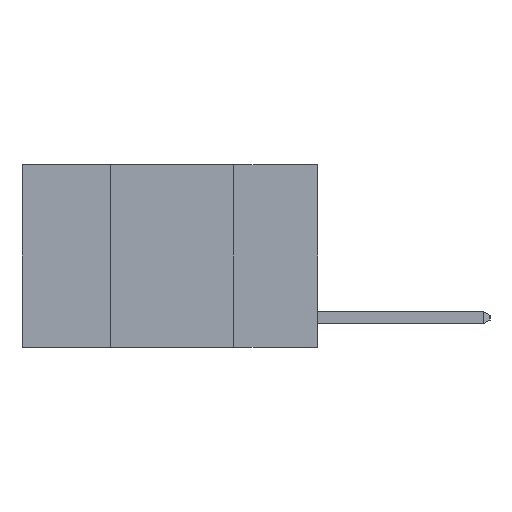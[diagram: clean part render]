
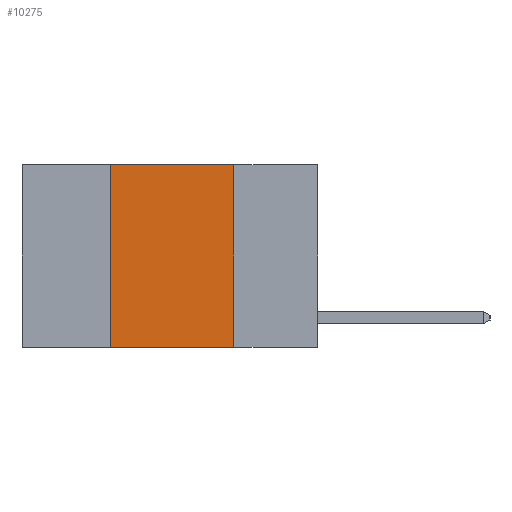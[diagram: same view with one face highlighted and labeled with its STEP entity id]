
A CAD part, left-side view. The second image highlights one B-rep face of the part: STEP entity #10275.
In plain terms, the highlighted planar face has unit normal (-1, 0, 0).
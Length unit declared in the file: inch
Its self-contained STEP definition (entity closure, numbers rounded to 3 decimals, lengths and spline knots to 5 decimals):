
#359 = DIRECTION ( 'NONE',  ( 0., 0., -1. ) ) ;
#1128 = DIRECTION ( 'NONE',  ( 0., -1., 0. ) ) ;
#1276 = LINE ( 'NONE', #9373, #3258 ) ;
#1300 = LINE ( 'NONE', #7426, #7578 ) ;
#1443 = ORIENTED_EDGE ( 'NONE', *, *, #9543, .F. ) ;
#1784 = LINE ( 'NONE', #6048, #2316 ) ;
#2316 = VECTOR ( 'NONE', #1128, 39.37008 ) ;
#2879 = CARTESIAN_POINT ( 'NONE',  ( 0., 0.6, 0. ) ) ;
#3106 = FACE_OUTER_BOUND ( 'NONE', #8566, .T. ) ;
#3258 = VECTOR ( 'NONE', #6106, 39.37008 ) ;
#3558 = VERTEX_POINT ( 'NONE', #8679 ) ;
#3678 = VERTEX_POINT ( 'NONE', #3871 ) ;
#3871 = CARTESIAN_POINT ( 'NONE',  ( 0., 0.17, 0. ) ) ;
#4033 = ORIENTED_EDGE ( 'NONE', *, *, #8474, .F. ) ;
#4898 = VERTEX_POINT ( 'NONE', #9851 ) ;
#4905 = CARTESIAN_POINT ( 'NONE',  ( 0., 0.17, 0. ) ) ;
#5311 = DIRECTION ( 'NONE',  ( 1., 0., 0. ) ) ;
#6048 = CARTESIAN_POINT ( 'NONE',  ( 0., 0.6, 0. ) ) ;
#6106 = DIRECTION ( 'NONE',  ( 0., 0., 1. ) ) ;
#6480 = ORIENTED_EDGE ( 'NONE', *, *, #6972, .T. ) ;
#6972 = EDGE_CURVE ( 'NONE', #4898, #9121, #1300, .T. ) ;
#7353 = ORIENTED_EDGE ( 'NONE', *, *, #9897, .F. ) ;
#7426 = CARTESIAN_POINT ( 'NONE',  ( 0., 0.6, -0.37 ) ) ;
#7578 = VECTOR ( 'NONE', #9889, 39.37008 ) ;
#8000 = CARTESIAN_POINT ( 'NONE',  ( 0., 0.17, -0.37 ) ) ;
#8336 = LINE ( 'NONE', #4905, #10506 ) ;
#8474 = EDGE_CURVE ( 'NONE', #4898, #3558, #1276, .T. ) ;
#8566 = EDGE_LOOP ( 'NONE', ( #7353, #1443, #4033, #6480 ) ) ;
#8614 = AXIS2_PLACEMENT_3D ( 'NONE', #2879, #5311, #359 ) ;
#8679 = CARTESIAN_POINT ( 'NONE',  ( 0., 0.42, 0. ) ) ;
#9121 = VERTEX_POINT ( 'NONE', #8000 ) ;
#9373 = CARTESIAN_POINT ( 'NONE',  ( 0., 0.42, 0. ) ) ;
#9543 = EDGE_CURVE ( 'NONE', #3558, #3678, #1784, .T. ) ;
#9851 = CARTESIAN_POINT ( 'NONE',  ( 0., 0.42, -0.37 ) ) ;
#9889 = DIRECTION ( 'NONE',  ( 0., -1., 0. ) ) ;
#9897 = EDGE_CURVE ( 'NONE', #3678, #9121, #8336, .T. ) ;
#10215 = PLANE ( 'NONE',  #8614 ) ;
#10275 = ADVANCED_FACE ( 'NONE', ( #3106 ), #10215, .F. ) ;
#10506 = VECTOR ( 'NONE', #10628, 39.37008 ) ;
#10628 = DIRECTION ( 'NONE',  ( 0., 0., -1. ) ) ;
